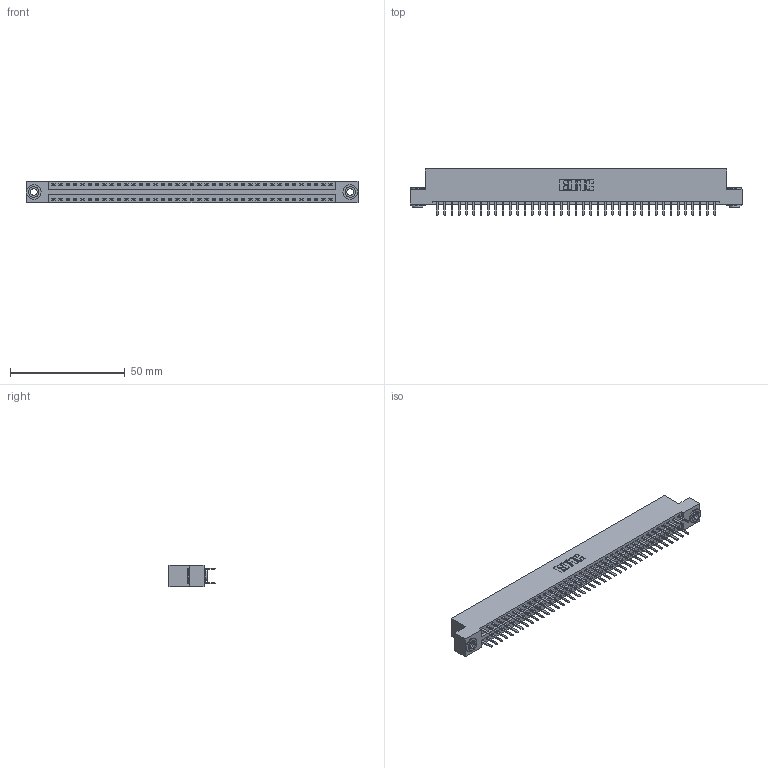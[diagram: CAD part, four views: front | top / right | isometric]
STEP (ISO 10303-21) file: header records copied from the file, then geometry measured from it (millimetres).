
FILE_DESCRIPTION (( 'STEP AP203' ), '1' );
FILE_NAME ('346-078-520-203.STEP', '2022-05-25T13:30:28', ( '' ), ( '' ), 'SwSTEP 2.0', 'SolidWorks 2020', '' );
FILE_SCHEMA (( 'CONFIG_CONTROL_DESIGN' ));
Length unit declared in the file: inch
Products named in the file (4): 345-292-001_345-293-120; 345-250-002_345-250-002-102; 346-078-520-203; 346 Part_Flush Mounting Lugs - 0.156 Dia-TH
Assembly tree (81 placements, depth 2):
  346-078-520-203
    346 Part_Flush Mounting Lugs - 0.156 Dia-TH
    345-292-001_345-293-120  x78
    345-250-002_345-250-002-102  x2
Bounding box: 144.4 x 20.02 x 9.4 mm (x, y, z)
Volume: 14024.4 mm3; surface area: 19398.7 mm2
Topology: 81 solids, 81 shells, 4542 faces, 13155 edges, 8558 vertices
Faces by surface type: plane 2986, cylinder 1548, cone 8
Entity records: 27036 total; most frequent: CARTESIAN_POINT 4453, ORIENTED_EDGE 4366, DIRECTION 3993, EDGE_CURVE 2183, LINE 1867, VECTOR 1867, VERTEX_POINT 1450, AXIS2_PLACEMENT_3D 1063
